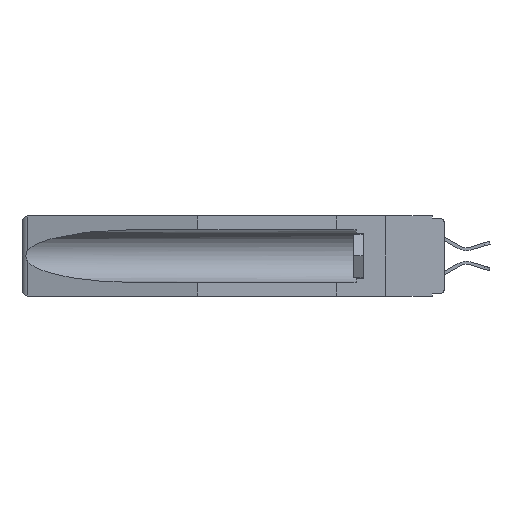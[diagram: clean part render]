
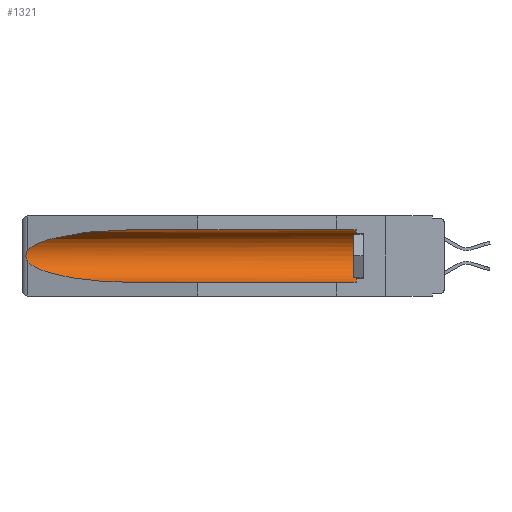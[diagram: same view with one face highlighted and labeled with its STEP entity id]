
A CAD part, left-side view. The second image highlights one B-rep face of the part: STEP entity #1321.
In plain terms, the highlighted cylindrical face has radius 2.857 mm (diameter 5.715 mm), a partial arc.
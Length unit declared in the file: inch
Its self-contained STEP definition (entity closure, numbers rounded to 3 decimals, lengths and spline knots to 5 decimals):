
#301 =( BOUNDED_CURVE ( )  B_SPLINE_CURVE ( 3, ( #10404, #2368, #2507, #976 ),
 .UNSPECIFIED., .F., .F. ) 
 B_SPLINE_CURVE_WITH_KNOTS ( ( 4, 4 ),
 ( 4.71239, 6.08839 ),
 .UNSPECIFIED. ) 
 CURVE ( )  GEOMETRIC_REPRESENTATION_ITEM ( )  RATIONAL_B_SPLINE_CURVE ( ( 1., 0.848, 0.848, 1. ) ) 
 REPRESENTATION_ITEM ( '' )  );
#407 = CARTESIAN_POINT ( 'NONE',  ( 0.25451, 1.48313, -0.24835 ) ) ;
#784 = DIRECTION ( 'NONE',  ( 0., 1., 0. ) ) ;
#976 = CARTESIAN_POINT ( 'NONE',  ( 0.26537, 1.52718, -0.14972 ) ) ;
#1201 = EDGE_CURVE ( 'NONE', #7051, #6467, #301, .T. ) ;
#1321 = ADVANCED_FACE ( 'NONE', ( #18364 ), #10553, .F. ) ;
#1642 = VERTEX_POINT ( 'NONE', #12840 ) ;
#1886 = CARTESIAN_POINT ( 'NONE',  ( 0.21114, 1.30732, -0.284 ) ) ;
#2368 = CARTESIAN_POINT ( 'NONE',  ( 0.21114, 1.30732, -0.059 ) ) ;
#2507 = CARTESIAN_POINT ( 'NONE',  ( 0.25451, 1.48313, -0.09465 ) ) ;
#2693 = CARTESIAN_POINT ( 'NONE',  ( 0.26537, 1.52718, -0.14972 ) ) ;
#3445 = CARTESIAN_POINT ( 'NONE',  ( 0.155, -0.30754, -0.059 ) ) ;
#3680 = ORIENTED_EDGE ( 'NONE', *, *, #16972, .T. ) ;
#4146 = ORIENTED_EDGE ( 'NONE', *, *, #1201, .T. ) ;
#4352 = CARTESIAN_POINT ( 'NONE',  ( 0.26597, 1.52961, -0.15275 ) ) ;
#4394 = DIRECTION ( 'NONE',  ( 0., 0., 1. ) ) ;
#4752 =( BOUNDED_CURVE ( )  B_SPLINE_CURVE ( 3, ( #16173, #407, #1886, #16376 ),
 .UNSPECIFIED., .F., .T. ) 
 B_SPLINE_CURVE_WITH_KNOTS ( ( 4, 4 ),
 ( 0.1948, 1.5708 ),
 .UNSPECIFIED. ) 
 CURVE ( )  GEOMETRIC_REPRESENTATION_ITEM ( )  RATIONAL_B_SPLINE_CURVE ( ( 1., 0.848, 0.848, 1. ) ) 
 REPRESENTATION_ITEM ( '' )  );
#5489 = EDGE_CURVE ( 'NONE', #1642, #16712, #12627, .T. ) ;
#6384 = AXIS2_PLACEMENT_3D ( 'NONE', #17042, #10632, #4394 ) ;
#6435 = ORIENTED_EDGE ( 'NONE', *, *, #12733, .T. ) ;
#6467 = VERTEX_POINT ( 'NONE', #2693 ) ;
#7051 = VERTEX_POINT ( 'NONE', #20268 ) ;
#7056 = EDGE_CURVE ( 'NONE', #1642, #20186, #19534, .T. ) ;
#7169 = CARTESIAN_POINT ( 'NONE',  ( 0.155, -0.30754, -0.284 ) ) ;
#8111 = DIRECTION ( 'NONE',  ( 0., 1., 0. ) ) ;
#8469 = CARTESIAN_POINT ( 'NONE',  ( 0.26655, 1.53094, -0.18657 ) ) ;
#8503 = B_SPLINE_CURVE_WITH_KNOTS ( 'NONE', 3,
 ( #9125, #4352, #10863, #16266, #10845, #17326, #9302, #8469, #13658, #18854 ),
 .UNSPECIFIED., .F., .F.,
 ( 4, 2, 2, 2, 4 ),
 ( 0., 0.00029, 0.00058, 0.00087, 0.00117 ),
 .UNSPECIFIED. ) ;
#9006 = CARTESIAN_POINT ( 'NONE',  ( 0.26537, 1.52718, -0.19328 ) ) ;
#9125 = CARTESIAN_POINT ( 'NONE',  ( 0.26537, 1.52718, -0.14972 ) ) ;
#9302 = CARTESIAN_POINT ( 'NONE',  ( 0.2673, 1.53269, -0.17917 ) ) ;
#10163 = VERTEX_POINT ( 'NONE', #9006 ) ;
#10404 = CARTESIAN_POINT ( 'NONE',  ( 0.155, 1.07973, -0.059 ) ) ;
#10457 = AXIS2_PLACEMENT_3D ( 'NONE', #18648, #10543, #12173 ) ;
#10543 = DIRECTION ( 'NONE',  ( 0., 1., 0. ) ) ;
#10553 = CYLINDRICAL_SURFACE ( 'NONE', #10457, 0.1125 ) ;
#10632 = DIRECTION ( 'NONE',  ( 0., -1., 0. ) ) ;
#10845 = CARTESIAN_POINT ( 'NONE',  ( 0.2675, 1.53308, -0.16763 ) ) ;
#10863 = CARTESIAN_POINT ( 'NONE',  ( 0.26654, 1.53092, -0.15636 ) ) ;
#12062 = CARTESIAN_POINT ( 'NONE',  ( 0.155, 0.126, -0.059 ) ) ;
#12173 = DIRECTION ( 'NONE',  ( 0., 0., 1. ) ) ;
#12627 = LINE ( 'NONE', #7169, #14148 ) ;
#12733 = EDGE_CURVE ( 'NONE', #20186, #7051, #15387, .T. ) ;
#12840 = CARTESIAN_POINT ( 'NONE',  ( 0.155, 0.126, -0.284 ) ) ;
#13658 = CARTESIAN_POINT ( 'NONE',  ( 0.26597, 1.5296, -0.19026 ) ) ;
#14148 = VECTOR ( 'NONE', #784, 39.37008 ) ;
#14968 = ORIENTED_EDGE ( 'NONE', *, *, #5489, .F. ) ;
#15387 = LINE ( 'NONE', #3445, #16373 ) ;
#16173 = CARTESIAN_POINT ( 'NONE',  ( 0.26537, 1.52718, -0.19328 ) ) ;
#16266 = CARTESIAN_POINT ( 'NONE',  ( 0.2673, 1.5327, -0.16383 ) ) ;
#16373 = VECTOR ( 'NONE', #8111, 39.37008 ) ;
#16376 = CARTESIAN_POINT ( 'NONE',  ( 0.155, 1.07973, -0.284 ) ) ;
#16575 = EDGE_LOOP ( 'NONE', ( #4146, #3680, #17361, #14968, #18287, #6435 ) ) ;
#16712 = VERTEX_POINT ( 'NONE', #18122 ) ;
#16972 = EDGE_CURVE ( 'NONE', #6467, #10163, #8503, .T. ) ;
#17042 = CARTESIAN_POINT ( 'NONE',  ( 0.155, 0.126, -0.1715 ) ) ;
#17326 = CARTESIAN_POINT ( 'NONE',  ( 0.2675, 1.53308, -0.17534 ) ) ;
#17361 = ORIENTED_EDGE ( 'NONE', *, *, #19366, .T. ) ;
#18122 = CARTESIAN_POINT ( 'NONE',  ( 0.155, 1.07973, -0.284 ) ) ;
#18287 = ORIENTED_EDGE ( 'NONE', *, *, #7056, .T. ) ;
#18364 = FACE_OUTER_BOUND ( 'NONE', #16575, .T. ) ;
#18648 = CARTESIAN_POINT ( 'NONE',  ( 0.155, -0.30754, -0.1715 ) ) ;
#18854 = CARTESIAN_POINT ( 'NONE',  ( 0.26537, 1.52718, -0.19328 ) ) ;
#19366 = EDGE_CURVE ( 'NONE', #10163, #16712, #4752, .T. ) ;
#19534 = CIRCLE ( 'NONE', #6384, 0.1125 ) ;
#20186 = VERTEX_POINT ( 'NONE', #12062 ) ;
#20268 = CARTESIAN_POINT ( 'NONE',  ( 0.155, 1.07973, -0.059 ) ) ;
